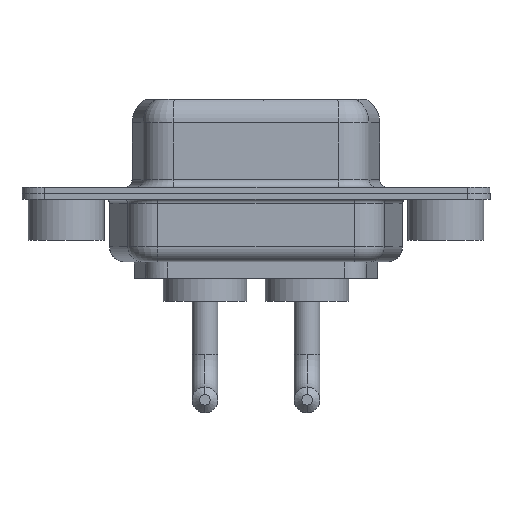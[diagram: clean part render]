
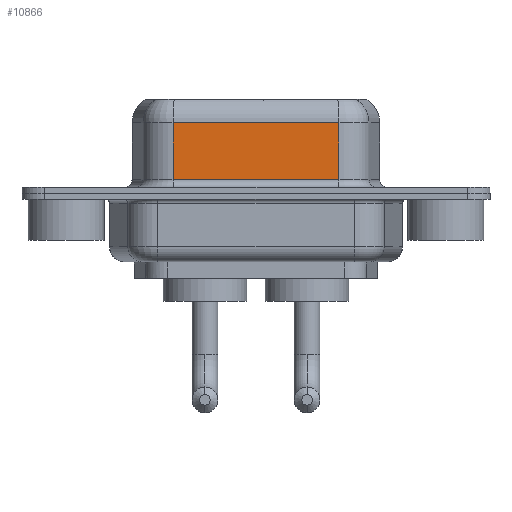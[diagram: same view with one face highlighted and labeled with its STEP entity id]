
A CAD part, front view. The second image highlights one B-rep face of the part: STEP entity #10866.
In plain terms, the highlighted planar face has unit normal (0, -1, 0).
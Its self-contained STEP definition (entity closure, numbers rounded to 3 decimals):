
#254 = AXIS2_PLACEMENT_3D ( 'NONE', #12856, #551, #2570 ) ;
#551 = DIRECTION ( 'NONE',  ( 0., 1., 0. ) ) ;
#560 = EDGE_CURVE ( 'NONE', #4081, #1275, #2282, .T. ) ;
#671 = CARTESIAN_POINT ( 'NONE',  ( 7.038, -3.95, 0.9 ) ) ;
#1275 = VERTEX_POINT ( 'NONE', #12491 ) ;
#1943 = VECTOR ( 'NONE', #5534, 1000. ) ;
#2158 = ORIENTED_EDGE ( 'NONE', *, *, #5520, .T. ) ;
#2282 = LINE ( 'NONE', #4394, #1943 ) ;
#2570 = DIRECTION ( 'NONE',  ( -1., 0., 0. ) ) ;
#3100 = LINE ( 'NONE', #10564, #12142 ) ;
#3703 = VECTOR ( 'NONE', #4549, 1000. ) ;
#4081 = VERTEX_POINT ( 'NONE', #671 ) ;
#4394 = CARTESIAN_POINT ( 'NONE',  ( 17.962, -3.95, 0.9 ) ) ;
#4549 = DIRECTION ( 'NONE',  ( 0., 0., -1. ) ) ;
#4680 = CARTESIAN_POINT ( 'NONE',  ( 7.038, -3.95, 6.4 ) ) ;
#4893 = VERTEX_POINT ( 'NONE', #8641 ) ;
#5404 = EDGE_LOOP ( 'NONE', ( #10978, #2158, #12588, #9696 ) ) ;
#5520 = EDGE_CURVE ( 'NONE', #12460, #4893, #12123, .T. ) ;
#5534 = DIRECTION ( 'NONE',  ( 1., 0., 0. ) ) ;
#5698 = LINE ( 'NONE', #4680, #3703 ) ;
#7459 = CARTESIAN_POINT ( 'NONE',  ( 17.962, -3.95, 4.65 ) ) ;
#8641 = CARTESIAN_POINT ( 'NONE',  ( 7.038, -3.95, 4.65 ) ) ;
#8828 = CARTESIAN_POINT ( 'NONE',  ( 17.962, -3.95, 4.65 ) ) ;
#9696 = ORIENTED_EDGE ( 'NONE', *, *, #560, .T. ) ;
#9771 = FACE_OUTER_BOUND ( 'NONE', #5404, .T. ) ;
#10564 = CARTESIAN_POINT ( 'NONE',  ( 17.962, -3.95, 6.4 ) ) ;
#10766 = EDGE_CURVE ( 'NONE', #4893, #4081, #5698, .T. ) ;
#10782 = PLANE ( 'NONE',  #254 ) ;
#10866 = ADVANCED_FACE ( 'NONE', ( #9771 ), #10782, .F. ) ;
#10978 = ORIENTED_EDGE ( 'NONE', *, *, #11074, .F. ) ;
#11074 = EDGE_CURVE ( 'NONE', #12460, #1275, #3100, .T. ) ;
#11511 = DIRECTION ( 'NONE',  ( 0., 0., -1. ) ) ;
#11858 = VECTOR ( 'NONE', #13365, 1000. ) ;
#12123 = LINE ( 'NONE', #8828, #11858 ) ;
#12142 = VECTOR ( 'NONE', #11511, 1000. ) ;
#12460 = VERTEX_POINT ( 'NONE', #7459 ) ;
#12491 = CARTESIAN_POINT ( 'NONE',  ( 17.962, -3.95, 0.9 ) ) ;
#12588 = ORIENTED_EDGE ( 'NONE', *, *, #10766, .T. ) ;
#12856 = CARTESIAN_POINT ( 'NONE',  ( 17.962, -3.95, 6.4 ) ) ;
#13365 = DIRECTION ( 'NONE',  ( -1., 0., 0. ) ) ;
